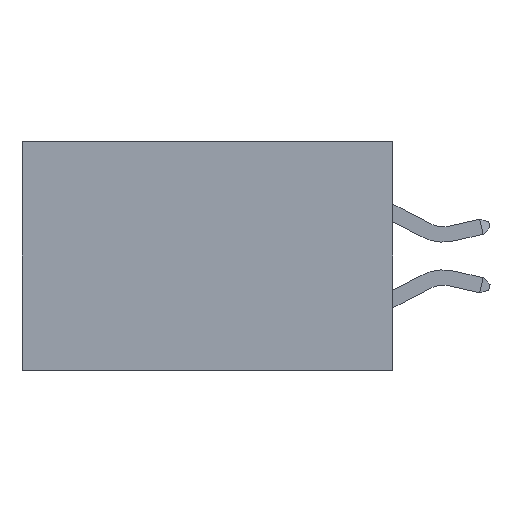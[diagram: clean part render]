
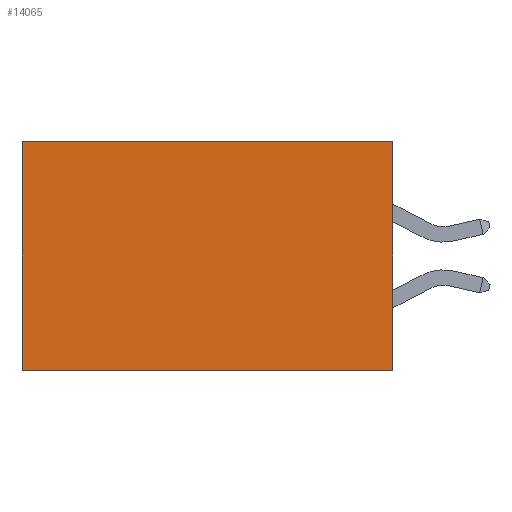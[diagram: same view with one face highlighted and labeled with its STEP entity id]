
A CAD part, left-side view. The second image highlights one B-rep face of the part: STEP entity #14065.
In plain terms, the highlighted planar face has unit normal (-1, 0, 0).
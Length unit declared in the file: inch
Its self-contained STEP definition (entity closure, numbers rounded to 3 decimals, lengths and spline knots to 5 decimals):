
#245 = CARTESIAN_POINT ( 'NONE',  ( 0.2875, 0., -0.37 ) ) ;
#1093 = CARTESIAN_POINT ( 'NONE',  ( 0.2875, 0.6, -0.37 ) ) ;
#2076 = VERTEX_POINT ( 'NONE', #18311 ) ;
#2189 = LINE ( 'NONE', #11433, #24324 ) ;
#3659 = CARTESIAN_POINT ( 'NONE',  ( 0.2875, 0.6, 0. ) ) ;
#4821 = EDGE_LOOP ( 'NONE', ( #16256, #5467, #27502, #10042 ) ) ;
#4877 = DIRECTION ( 'NONE',  ( 0., 0., -1. ) ) ;
#5467 = ORIENTED_EDGE ( 'NONE', *, *, #21224, .F. ) ;
#8798 = VERTEX_POINT ( 'NONE', #1093 ) ;
#9062 = PLANE ( 'NONE',  #16455 ) ;
#9516 = EDGE_CURVE ( 'NONE', #2076, #17678, #12585, .T. ) ;
#10042 = ORIENTED_EDGE ( 'NONE', *, *, #27673, .T. ) ;
#10643 = DIRECTION ( 'NONE',  ( 0., 0., -1. ) ) ;
#11067 = DIRECTION ( 'NONE',  ( 1., 0., 0. ) ) ;
#11433 = CARTESIAN_POINT ( 'NONE',  ( 0.2875, 0., 0. ) ) ;
#12585 = LINE ( 'NONE', #13821, #19262 ) ;
#12801 = DIRECTION ( 'NONE',  ( 0., 1., 0. ) ) ;
#13605 = CARTESIAN_POINT ( 'NONE',  ( 0.2875, 0., 0. ) ) ;
#13821 = CARTESIAN_POINT ( 'NONE',  ( 0.2875, 0., 0. ) ) ;
#14065 = ADVANCED_FACE ( 'NONE', ( #26689 ), #9062, .F. ) ;
#15081 = VECTOR ( 'NONE', #12801, 39.37008 ) ;
#16256 = ORIENTED_EDGE ( 'NONE', *, *, #21211, .T. ) ;
#16455 = AXIS2_PLACEMENT_3D ( 'NONE', #13605, #11067, #20082 ) ;
#17678 = VERTEX_POINT ( 'NONE', #245 ) ;
#18311 = CARTESIAN_POINT ( 'NONE',  ( 0.2875, 0., 0. ) ) ;
#19262 = VECTOR ( 'NONE', #4877, 39.37008 ) ;
#19275 = CARTESIAN_POINT ( 'NONE',  ( 0.2875, 0., -0.37 ) ) ;
#19955 = LINE ( 'NONE', #19275, #15081 ) ;
#20082 = DIRECTION ( 'NONE',  ( 0., 0., -1. ) ) ;
#20464 = DIRECTION ( 'NONE',  ( 0., 1., 0. ) ) ;
#21211 = EDGE_CURVE ( 'NONE', #27160, #8798, #25917, .T. ) ;
#21224 = EDGE_CURVE ( 'NONE', #17678, #8798, #19955, .T. ) ;
#21891 = CARTESIAN_POINT ( 'NONE',  ( 0.2875, 0.6, 0. ) ) ;
#24324 = VECTOR ( 'NONE', #20464, 39.37008 ) ;
#25917 = LINE ( 'NONE', #3659, #27287 ) ;
#26689 = FACE_OUTER_BOUND ( 'NONE', #4821, .T. ) ;
#27160 = VERTEX_POINT ( 'NONE', #21891 ) ;
#27287 = VECTOR ( 'NONE', #10643, 39.37008 ) ;
#27502 = ORIENTED_EDGE ( 'NONE', *, *, #9516, .F. ) ;
#27673 = EDGE_CURVE ( 'NONE', #2076, #27160, #2189, .T. ) ;
